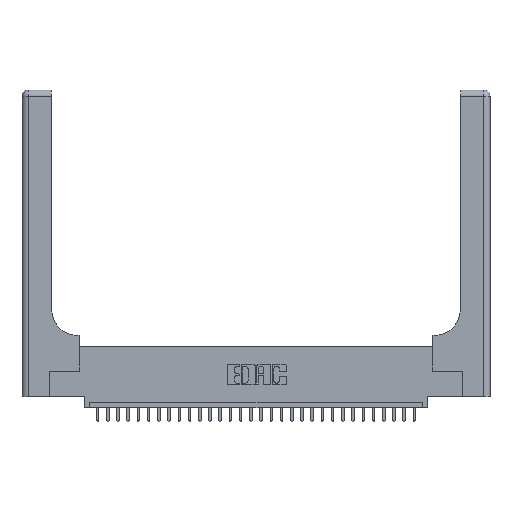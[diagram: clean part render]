
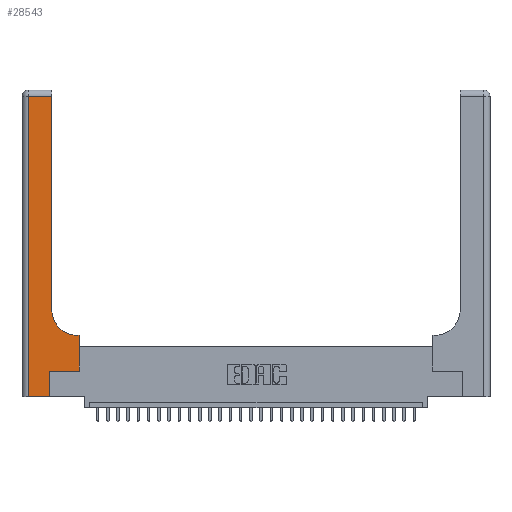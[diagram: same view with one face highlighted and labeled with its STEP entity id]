
A CAD part, top view. The second image highlights one B-rep face of the part: STEP entity #28543.
In plain terms, the highlighted planar face has unit normal (0, 0, 1).
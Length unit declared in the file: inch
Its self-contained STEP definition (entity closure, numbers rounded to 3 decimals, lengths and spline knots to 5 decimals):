
#377 = CARTESIAN_POINT ( 'NONE',  ( 0.269, 0., 0.37 ) ) ;
#1082 = LINE ( 'NONE', #8024, #30424 ) ;
#1133 = VERTEX_POINT ( 'NONE', #377 ) ;
#1474 = DIRECTION ( 'NONE',  ( 0., 1., 0. ) ) ;
#1599 = CARTESIAN_POINT ( 'NONE',  ( 0.269, 0.25, 0.37 ) ) ;
#1724 = CARTESIAN_POINT ( 'NONE',  ( 0.06, 0., 0.37 ) ) ;
#1893 = PLANE ( 'NONE',  #4245 ) ;
#2091 = DIRECTION ( 'NONE',  ( -1., 0., 0. ) ) ;
#2387 = VECTOR ( 'NONE', #9171, 39.37008 ) ;
#2602 = EDGE_CURVE ( 'NONE', #1133, #4620, #13965, .T. ) ;
#3805 = LINE ( 'NONE', #11058, #23520 ) ;
#4245 = AXIS2_PLACEMENT_3D ( 'NONE', #25675, #28148, #2091 ) ;
#4620 = VERTEX_POINT ( 'NONE', #1599 ) ;
#5552 = CARTESIAN_POINT ( 'NONE',  ( 0.269, 0., 0.37 ) ) ;
#6129 = CARTESIAN_POINT ( 'NONE',  ( 0.06, 3., 0.37 ) ) ;
#6401 = LINE ( 'NONE', #20525, #13105 ) ;
#6815 = DIRECTION ( 'NONE',  ( -1., 0., 0. ) ) ;
#8024 = CARTESIAN_POINT ( 'NONE',  ( 0.2915, 0.6, 0.37 ) ) ;
#8404 = VERTEX_POINT ( 'NONE', #24377 ) ;
#8798 = ORIENTED_EDGE ( 'NONE', *, *, #11495, .T. ) ;
#9171 = DIRECTION ( 'NONE',  ( 1., 0., 0. ) ) ;
#9409 = CIRCLE ( 'NONE', #14962, 0.25 ) ;
#9540 = VECTOR ( 'NONE', #27212, 39.37008 ) ;
#9832 = LINE ( 'NONE', #11442, #2387 ) ;
#10382 = VERTEX_POINT ( 'NONE', #24084 ) ;
#10689 = CARTESIAN_POINT ( 'NONE',  ( 0.269, 0.25, 0.37 ) ) ;
#11058 = CARTESIAN_POINT ( 'NONE',  ( 0.5585, 0.25, 0.37 ) ) ;
#11202 = EDGE_CURVE ( 'NONE', #10382, #30483, #9409, .T. ) ;
#11442 = CARTESIAN_POINT ( 'NONE',  ( 0., 0., 0.37 ) ) ;
#11495 = EDGE_CURVE ( 'NONE', #30483, #28916, #6401, .T. ) ;
#11516 = LINE ( 'NONE', #27740, #18192 ) ;
#11749 = VERTEX_POINT ( 'NONE', #21238 ) ;
#12889 = VERTEX_POINT ( 'NONE', #1724 ) ;
#13105 = VECTOR ( 'NONE', #1474, 39.37008 ) ;
#13965 = LINE ( 'NONE', #5552, #9540 ) ;
#14390 = VECTOR ( 'NONE', #20675, 39.37008 ) ;
#14391 = EDGE_CURVE ( 'NONE', #11749, #12889, #24115, .T. ) ;
#14962 = AXIS2_PLACEMENT_3D ( 'NONE', #18165, #20384, #22744 ) ;
#15873 = LINE ( 'NONE', #10689, #14390 ) ;
#16044 = ORIENTED_EDGE ( 'NONE', *, *, #21043, .T. ) ;
#18165 = CARTESIAN_POINT ( 'NONE',  ( 0.5415, 0.85, 0.37 ) ) ;
#18192 = VECTOR ( 'NONE', #6815, 39.37008 ) ;
#18286 = ORIENTED_EDGE ( 'NONE', *, *, #2602, .T. ) ;
#18740 = VERTEX_POINT ( 'NONE', #20895 ) ;
#19851 = DIRECTION ( 'NONE',  ( 0., 1., 0. ) ) ;
#20384 = DIRECTION ( 'NONE',  ( 0., 0., -1. ) ) ;
#20466 = DIRECTION ( 'NONE',  ( 0., -1., 0. ) ) ;
#20525 = CARTESIAN_POINT ( 'NONE',  ( 0.2915, 3., 0.37 ) ) ;
#20675 = DIRECTION ( 'NONE',  ( 1., 0., 0. ) ) ;
#20721 = EDGE_LOOP ( 'NONE', ( #8798, #29922, #25837, #16044, #18286, #28823, #26636, #23040, #29573 ) ) ;
#20895 = CARTESIAN_POINT ( 'NONE',  ( 0.5585, 0.6, 0.37 ) ) ;
#21043 = EDGE_CURVE ( 'NONE', #12889, #1133, #9832, .T. ) ;
#21238 = CARTESIAN_POINT ( 'NONE',  ( 0.06, 2.94, 0.37 ) ) ;
#22291 = EDGE_CURVE ( 'NONE', #4620, #8404, #15873, .T. ) ;
#22744 = DIRECTION ( 'NONE',  ( 1., 0., 0. ) ) ;
#23040 = ORIENTED_EDGE ( 'NONE', *, *, #26129, .T. ) ;
#23145 = EDGE_CURVE ( 'NONE', #8404, #18740, #3805, .T. ) ;
#23216 = FACE_OUTER_BOUND ( 'NONE', #20721, .T. ) ;
#23520 = VECTOR ( 'NONE', #19851, 39.37008 ) ;
#24031 = CARTESIAN_POINT ( 'NONE',  ( 0.2915, 0.85, 0.37 ) ) ;
#24084 = CARTESIAN_POINT ( 'NONE',  ( 0.5415, 0.6, 0.37 ) ) ;
#24115 = LINE ( 'NONE', #6129, #27406 ) ;
#24377 = CARTESIAN_POINT ( 'NONE',  ( 0.5585, 0.25, 0.37 ) ) ;
#24594 = DIRECTION ( 'NONE',  ( -1., 0., 0. ) ) ;
#25025 = EDGE_CURVE ( 'NONE', #28916, #11749, #11516, .T. ) ;
#25675 = CARTESIAN_POINT ( 'NONE',  ( 0., 3., 0.37 ) ) ;
#25837 = ORIENTED_EDGE ( 'NONE', *, *, #14391, .T. ) ;
#26129 = EDGE_CURVE ( 'NONE', #18740, #10382, #1082, .T. ) ;
#26636 = ORIENTED_EDGE ( 'NONE', *, *, #23145, .T. ) ;
#27212 = DIRECTION ( 'NONE',  ( 0., 1., 0. ) ) ;
#27406 = VECTOR ( 'NONE', #20466, 39.37008 ) ;
#27740 = CARTESIAN_POINT ( 'NONE',  ( 0., 2.94, 0.37 ) ) ;
#28148 = DIRECTION ( 'NONE',  ( 0., 0., -1. ) ) ;
#28543 = ADVANCED_FACE ( 'NONE', ( #23216 ), #1893, .F. ) ;
#28823 = ORIENTED_EDGE ( 'NONE', *, *, #22291, .T. ) ;
#28916 = VERTEX_POINT ( 'NONE', #29289 ) ;
#29289 = CARTESIAN_POINT ( 'NONE',  ( 0.2915, 2.94, 0.37 ) ) ;
#29573 = ORIENTED_EDGE ( 'NONE', *, *, #11202, .T. ) ;
#29922 = ORIENTED_EDGE ( 'NONE', *, *, #25025, .T. ) ;
#30424 = VECTOR ( 'NONE', #24594, 39.37008 ) ;
#30483 = VERTEX_POINT ( 'NONE', #24031 ) ;
